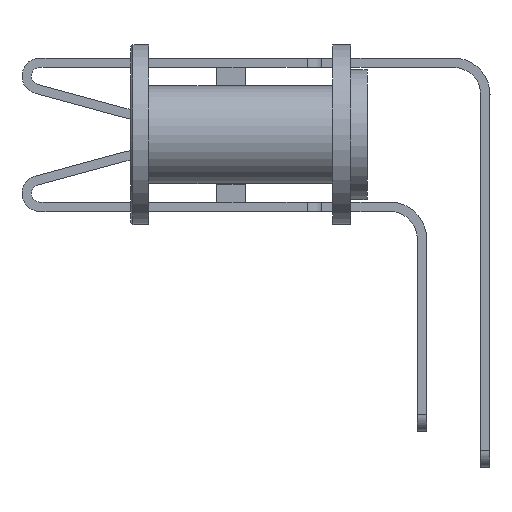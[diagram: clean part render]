
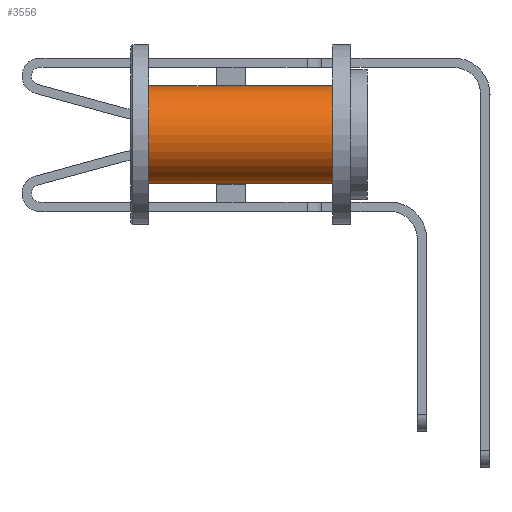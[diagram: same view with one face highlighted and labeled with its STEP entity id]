
A CAD part, left-side view. The second image highlights one B-rep face of the part: STEP entity #3556.
In plain terms, the highlighted cylindrical face has radius 1.727 mm (diameter 3.454 mm), a partial arc.
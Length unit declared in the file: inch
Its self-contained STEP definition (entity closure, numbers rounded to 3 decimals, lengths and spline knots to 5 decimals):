
#206 = FACE_OUTER_BOUND ( 'NONE', #25676, .T. ) ;
#1125 = AXIS2_PLACEMENT_3D ( 'NONE', #30447, #25419, #5738 ) ;
#1673 = CARTESIAN_POINT ( 'NONE',  ( 0., 0.28, 0.068 ) ) ;
#1711 = DIRECTION ( 'NONE',  ( 0., 1., 0. ) ) ;
#1878 = CARTESIAN_POINT ( 'NONE',  ( 0., 0.025, 0. ) ) ;
#3556 = ADVANCED_FACE ( 'NONE', ( #206 ), #30782, .T. ) ;
#3719 = CARTESIAN_POINT ( 'NONE',  ( 0., 0.025, -0.068 ) ) ;
#4139 = DIRECTION ( 'NONE',  ( 0., -1., 0. ) ) ;
#5247 = CIRCLE ( 'NONE', #11644, 0.068 ) ;
#5738 = DIRECTION ( 'NONE',  ( 0., 0., -1. ) ) ;
#5988 = AXIS2_PLACEMENT_3D ( 'NONE', #1878, #1711, #32422 ) ;
#8132 = CIRCLE ( 'NONE', #5988, 0.068 ) ;
#11644 = AXIS2_PLACEMENT_3D ( 'NONE', #28754, #23411, #20915 ) ;
#11895 = VECTOR ( 'NONE', #4139, 39.37008 ) ;
#11978 = LINE ( 'NONE', #26821, #11895 ) ;
#12868 = VERTEX_POINT ( 'NONE', #1673 ) ;
#13892 = ORIENTED_EDGE ( 'NONE', *, *, #31515, .F. ) ;
#13941 = EDGE_CURVE ( 'NONE', #30819, #14129, #20082, .T. ) ;
#14129 = VERTEX_POINT ( 'NONE', #3719 ) ;
#16120 = ORIENTED_EDGE ( 'NONE', *, *, #13941, .T. ) ;
#20082 = LINE ( 'NONE', #30267, #30867 ) ;
#20915 = DIRECTION ( 'NONE',  ( 0., 0., 1. ) ) ;
#21853 = EDGE_CURVE ( 'NONE', #14129, #27260, #8132, .T. ) ;
#22196 = CARTESIAN_POINT ( 'NONE',  ( 0., 0.28, -0.068 ) ) ;
#22902 = ORIENTED_EDGE ( 'NONE', *, *, #32662, .F. ) ;
#23411 = DIRECTION ( 'NONE',  ( 0., 1., 0. ) ) ;
#25419 = DIRECTION ( 'NONE',  ( 0., -1., 0. ) ) ;
#25676 = EDGE_LOOP ( 'NONE', ( #22902, #13892, #16120, #28775 ) ) ;
#26821 = CARTESIAN_POINT ( 'NONE',  ( 0., 0.328, 0.068 ) ) ;
#27260 = VERTEX_POINT ( 'NONE', #28589 ) ;
#28589 = CARTESIAN_POINT ( 'NONE',  ( 0., 0.025, 0.068 ) ) ;
#28754 = CARTESIAN_POINT ( 'NONE',  ( 0., 0.28, 0. ) ) ;
#28775 = ORIENTED_EDGE ( 'NONE', *, *, #21853, .T. ) ;
#30267 = CARTESIAN_POINT ( 'NONE',  ( 0., 0.328, -0.068 ) ) ;
#30447 = CARTESIAN_POINT ( 'NONE',  ( 0., 0.328, 0. ) ) ;
#30782 = CYLINDRICAL_SURFACE ( 'NONE', #1125, 0.068 ) ;
#30819 = VERTEX_POINT ( 'NONE', #22196 ) ;
#30867 = VECTOR ( 'NONE', #32594, 39.37008 ) ;
#31515 = EDGE_CURVE ( 'NONE', #30819, #12868, #5247, .T. ) ;
#32422 = DIRECTION ( 'NONE',  ( 0., 0., 1. ) ) ;
#32594 = DIRECTION ( 'NONE',  ( 0., -1., 0. ) ) ;
#32662 = EDGE_CURVE ( 'NONE', #12868, #27260, #11978, .T. ) ;
